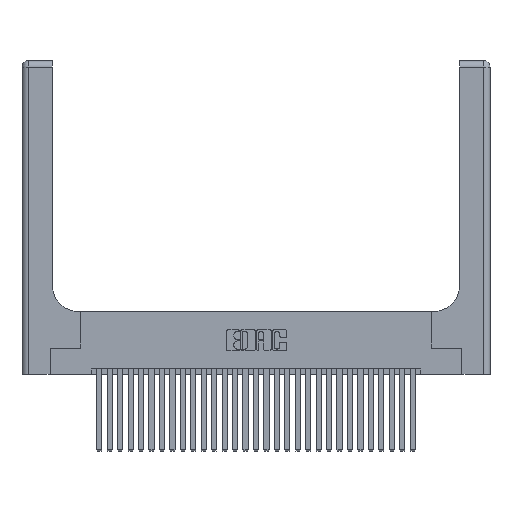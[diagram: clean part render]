
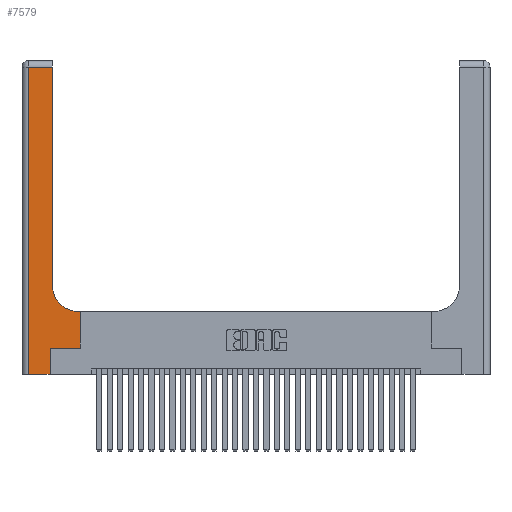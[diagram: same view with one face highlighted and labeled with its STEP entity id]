
A CAD part, top view. The second image highlights one B-rep face of the part: STEP entity #7579.
In plain terms, the highlighted planar face has unit normal (0, 0, 1).
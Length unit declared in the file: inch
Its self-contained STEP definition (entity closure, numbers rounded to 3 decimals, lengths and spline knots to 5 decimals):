
#62 = DIRECTION ( 'NONE',  ( 1., 0., 0. ) ) ;
#128 = LINE ( 'NONE', #16248, #25438 ) ;
#263 = CARTESIAN_POINT ( 'NONE',  ( 0.5415, 0.85, 0.37 ) ) ;
#872 = CARTESIAN_POINT ( 'NONE',  ( 0., 3., 0.37 ) ) ;
#1028 = VECTOR ( 'NONE', #23272, 39.37008 ) ;
#1040 = ORIENTED_EDGE ( 'NONE', *, *, #29772, .T. ) ;
#1516 = EDGE_CURVE ( 'NONE', #13073, #20919, #128, .T. ) ;
#1625 = ORIENTED_EDGE ( 'NONE', *, *, #27316, .T. ) ;
#1686 = VERTEX_POINT ( 'NONE', #6691 ) ;
#2325 = CARTESIAN_POINT ( 'NONE',  ( 0., 0., 0.37 ) ) ;
#2335 = EDGE_CURVE ( 'NONE', #11111, #22625, #13020, .T. ) ;
#2345 = ORIENTED_EDGE ( 'NONE', *, *, #2335, .T. ) ;
#3077 = LINE ( 'NONE', #2325, #12047 ) ;
#3519 = CARTESIAN_POINT ( 'NONE',  ( 0.5585, 0.25, 0.37 ) ) ;
#4955 = DIRECTION ( 'NONE',  ( 1., 0., 0. ) ) ;
#5193 = ORIENTED_EDGE ( 'NONE', *, *, #1516, .T. ) ;
#5295 = LINE ( 'NONE', #26286, #26132 ) ;
#6042 = CARTESIAN_POINT ( 'NONE',  ( 0.06, 3., 0.37 ) ) ;
#6083 = AXIS2_PLACEMENT_3D ( 'NONE', #263, #9861, #4955 ) ;
#6279 = DIRECTION ( 'NONE',  ( 0., 1., 0. ) ) ;
#6468 = ORIENTED_EDGE ( 'NONE', *, *, #19363, .T. ) ;
#6470 = DIRECTION ( 'NONE',  ( 0., 1., 0. ) ) ;
#6691 = CARTESIAN_POINT ( 'NONE',  ( 0.06, 2.94, 0.37 ) ) ;
#6804 = CARTESIAN_POINT ( 'NONE',  ( 0.269, 0.25, 0.37 ) ) ;
#6878 = VERTEX_POINT ( 'NONE', #24301 ) ;
#7579 = ADVANCED_FACE ( 'NONE', ( #13494 ), #13186, .F. ) ;
#7585 = DIRECTION ( 'NONE',  ( 0., 1., 0. ) ) ;
#7780 = CARTESIAN_POINT ( 'NONE',  ( 0., 2.94, 0.37 ) ) ;
#7854 = VECTOR ( 'NONE', #13222, 39.37008 ) ;
#8350 = EDGE_LOOP ( 'NONE', ( #1040, #6468, #11848, #1625, #9670, #5193, #15991, #28547, #2345 ) ) ;
#8485 = VECTOR ( 'NONE', #6279, 39.37008 ) ;
#8730 = EDGE_CURVE ( 'NONE', #1686, #19606, #20875, .T. ) ;
#9659 = CARTESIAN_POINT ( 'NONE',  ( 0.06, 0., 0.37 ) ) ;
#9670 = ORIENTED_EDGE ( 'NONE', *, *, #19507, .T. ) ;
#9861 = DIRECTION ( 'NONE',  ( 0., 0., -1. ) ) ;
#10283 = VERTEX_POINT ( 'NONE', #10569 ) ;
#10520 = LINE ( 'NONE', #7780, #29857 ) ;
#10569 = CARTESIAN_POINT ( 'NONE',  ( 0.269, 0., 0.37 ) ) ;
#11111 = VERTEX_POINT ( 'NONE', #25701 ) ;
#11848 = ORIENTED_EDGE ( 'NONE', *, *, #8730, .T. ) ;
#12047 = VECTOR ( 'NONE', #62, 39.37008 ) ;
#12655 = DIRECTION ( 'NONE',  ( -1., 0., 0. ) ) ;
#13020 = CIRCLE ( 'NONE', #6083, 0.25 ) ;
#13073 = VERTEX_POINT ( 'NONE', #6804 ) ;
#13186 = PLANE ( 'NONE',  #18370 ) ;
#13222 = DIRECTION ( 'NONE',  ( 0., -1., 0. ) ) ;
#13494 = FACE_OUTER_BOUND ( 'NONE', #8350, .T. ) ;
#13706 = LINE ( 'NONE', #18138, #8485 ) ;
#13816 = LINE ( 'NONE', #20824, #16047 ) ;
#14846 = LINE ( 'NONE', #20686, #1028 ) ;
#15260 = DIRECTION ( 'NONE',  ( 0., 0., -1. ) ) ;
#15991 = ORIENTED_EDGE ( 'NONE', *, *, #22163, .T. ) ;
#16047 = VECTOR ( 'NONE', #6470, 39.37008 ) ;
#16248 = CARTESIAN_POINT ( 'NONE',  ( 0.269, 0.25, 0.37 ) ) ;
#18138 = CARTESIAN_POINT ( 'NONE',  ( 0.5585, 0.25, 0.37 ) ) ;
#18370 = AXIS2_PLACEMENT_3D ( 'NONE', #872, #15260, #22532 ) ;
#19363 = EDGE_CURVE ( 'NONE', #6878, #1686, #10520, .T. ) ;
#19507 = EDGE_CURVE ( 'NONE', #10283, #13073, #5295, .T. ) ;
#19606 = VERTEX_POINT ( 'NONE', #9659 ) ;
#20063 = VERTEX_POINT ( 'NONE', #28354 ) ;
#20686 = CARTESIAN_POINT ( 'NONE',  ( 0.2915, 0.6, 0.37 ) ) ;
#20824 = CARTESIAN_POINT ( 'NONE',  ( 0.2915, 3., 0.37 ) ) ;
#20875 = LINE ( 'NONE', #6042, #7854 ) ;
#20919 = VERTEX_POINT ( 'NONE', #3519 ) ;
#22163 = EDGE_CURVE ( 'NONE', #20919, #20063, #13706, .T. ) ;
#22532 = DIRECTION ( 'NONE',  ( -1., 0., 0. ) ) ;
#22625 = VERTEX_POINT ( 'NONE', #27497 ) ;
#23272 = DIRECTION ( 'NONE',  ( -1., 0., 0. ) ) ;
#24055 = EDGE_CURVE ( 'NONE', #20063, #11111, #14846, .T. ) ;
#24301 = CARTESIAN_POINT ( 'NONE',  ( 0.2915, 2.94, 0.37 ) ) ;
#25438 = VECTOR ( 'NONE', #30617, 39.37008 ) ;
#25701 = CARTESIAN_POINT ( 'NONE',  ( 0.5415, 0.6, 0.37 ) ) ;
#26132 = VECTOR ( 'NONE', #7585, 39.37008 ) ;
#26286 = CARTESIAN_POINT ( 'NONE',  ( 0.269, 0., 0.37 ) ) ;
#27316 = EDGE_CURVE ( 'NONE', #19606, #10283, #3077, .T. ) ;
#27497 = CARTESIAN_POINT ( 'NONE',  ( 0.2915, 0.85, 0.37 ) ) ;
#28354 = CARTESIAN_POINT ( 'NONE',  ( 0.5585, 0.6, 0.37 ) ) ;
#28547 = ORIENTED_EDGE ( 'NONE', *, *, #24055, .T. ) ;
#29772 = EDGE_CURVE ( 'NONE', #22625, #6878, #13816, .T. ) ;
#29857 = VECTOR ( 'NONE', #12655, 39.37008 ) ;
#30617 = DIRECTION ( 'NONE',  ( 1., 0., 0. ) ) ;
